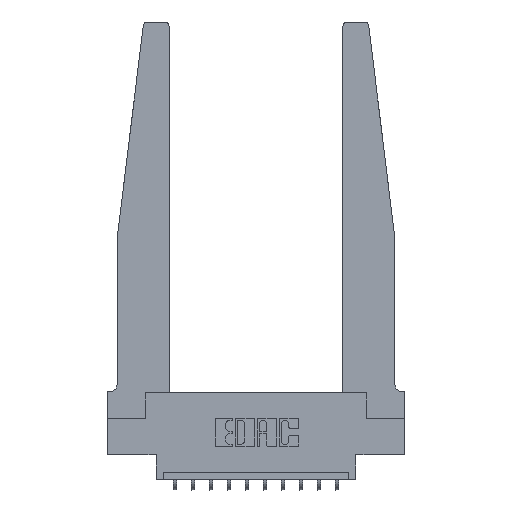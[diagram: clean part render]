
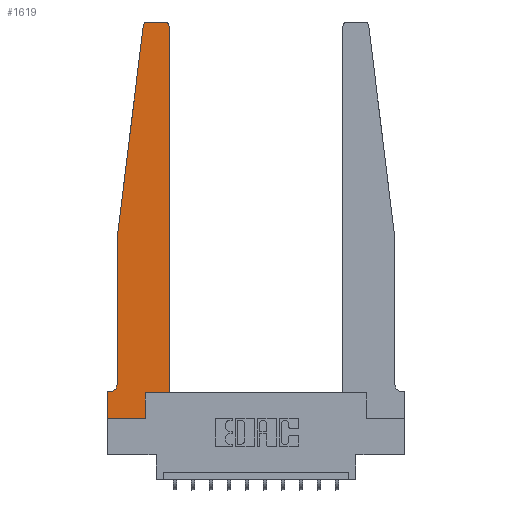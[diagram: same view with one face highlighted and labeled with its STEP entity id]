
A CAD part, top view. The second image highlights one B-rep face of the part: STEP entity #1619.
In plain terms, the highlighted planar face has unit normal (0, 0, 1).
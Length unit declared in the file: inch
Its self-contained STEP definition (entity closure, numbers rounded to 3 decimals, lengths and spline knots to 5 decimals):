
#219 = CARTESIAN_POINT ( 'NONE',  ( 0.015, 0.1875, 0.37 ) ) ;
#245 = DIRECTION ( 'NONE',  ( 0., 0., -1. ) ) ;
#351 = CARTESIAN_POINT ( 'NONE',  ( 0., 0.1875, 0.37 ) ) ;
#1283 = LINE ( 'NONE', #11136, #10915 ) ;
#1291 = VECTOR ( 'NONE', #9293, 39.37008 ) ;
#1331 = VERTEX_POINT ( 'NONE', #351 ) ;
#1425 = CARTESIAN_POINT ( 'NONE',  ( 0.065, 0.2375, 0.37 ) ) ;
#1446 = DIRECTION ( 'NONE',  ( -1., 0., 0. ) ) ;
#1536 = CARTESIAN_POINT ( 'NONE',  ( 0.425, 0.18, 0.37 ) ) ;
#1566 = DIRECTION ( 'NONE',  ( 0., 0., 1. ) ) ;
#1619 = ADVANCED_FACE ( 'NONE', ( #9924 ), #7503, .T. ) ;
#1737 = ORIENTED_EDGE ( 'NONE', *, *, #12814, .T. ) ;
#1752 = EDGE_CURVE ( 'NONE', #1331, #8008, #2641, .T. ) ;
#1868 = CARTESIAN_POINT ( 'NONE',  ( 0.065, 0.1875, 0.37 ) ) ;
#2068 = AXIS2_PLACEMENT_3D ( 'NONE', #9956, #1566, #6478 ) ;
#2637 = DIRECTION ( 'NONE',  ( 0., 1., 0. ) ) ;
#2641 = LINE ( 'NONE', #12758, #14164 ) ;
#2652 = LINE ( 'NONE', #6215, #13630 ) ;
#2748 = ORIENTED_EDGE ( 'NONE', *, *, #3446, .T. ) ;
#2854 = VECTOR ( 'NONE', #7429, 39.37008 ) ;
#2902 = CIRCLE ( 'NONE', #13999, 0.03 ) ;
#2942 = CARTESIAN_POINT ( 'NONE',  ( 0.2605, 0., 0.37 ) ) ;
#3031 = VERTEX_POINT ( 'NONE', #15523 ) ;
#3446 = EDGE_CURVE ( 'NONE', #14721, #13834, #15657, .T. ) ;
#3712 = CARTESIAN_POINT ( 'NONE',  ( 0., 0., 0.37 ) ) ;
#4086 = DIRECTION ( 'NONE',  ( -1., 0., 0. ) ) ;
#4157 = VECTOR ( 'NONE', #8885, 39.37008 ) ;
#4207 = EDGE_CURVE ( 'NONE', #13834, #12149, #9402, .T. ) ;
#4646 = CARTESIAN_POINT ( 'NONE',  ( 0.2605, 0.18, 0.37 ) ) ;
#4832 = DIRECTION ( 'NONE',  ( 1., 0., 0. ) ) ;
#4984 = DIRECTION ( 'NONE',  ( 1., 0., 0. ) ) ;
#5089 = EDGE_CURVE ( 'NONE', #6378, #12727, #10977, .T. ) ;
#5224 = CARTESIAN_POINT ( 'NONE',  ( 0.065, 1.25, 0.37 ) ) ;
#5264 = DIRECTION ( 'NONE',  ( 1., 0., 0. ) ) ;
#5334 = EDGE_CURVE ( 'NONE', #3031, #5651, #10321, .T. ) ;
#5345 = CARTESIAN_POINT ( 'NONE',  ( 0.395, 2.72, 0.37 ) ) ;
#5479 = LINE ( 'NONE', #7670, #4157 ) ;
#5651 = VERTEX_POINT ( 'NONE', #10226 ) ;
#5685 = CARTESIAN_POINT ( 'NONE',  ( 0.24675, 2.72367, 0.37 ) ) ;
#6155 = EDGE_LOOP ( 'NONE', ( #14824, #12152, #13387, #2748, #9065, #15544, #7193, #8934, #7471, #1737, #7129, #10539 ) ) ;
#6215 = CARTESIAN_POINT ( 'NONE',  ( 0.065, 1.25, 0.37 ) ) ;
#6341 = VECTOR ( 'NONE', #2637, 39.37008 ) ;
#6378 = VERTEX_POINT ( 'NONE', #13663 ) ;
#6478 = DIRECTION ( 'NONE',  ( 1., 0., 0. ) ) ;
#6559 = EDGE_CURVE ( 'NONE', #12727, #3031, #2902, .T. ) ;
#6861 = LINE ( 'NONE', #1868, #1291 ) ;
#6907 = EDGE_CURVE ( 'NONE', #15174, #8755, #5479, .T. ) ;
#6957 = CARTESIAN_POINT ( 'NONE',  ( 0.065, 1.25, 0.37 ) ) ;
#7062 = AXIS2_PLACEMENT_3D ( 'NONE', #7827, #245, #1446 ) ;
#7129 = ORIENTED_EDGE ( 'NONE', *, *, #5089, .T. ) ;
#7193 = ORIENTED_EDGE ( 'NONE', *, *, #1752, .T. ) ;
#7429 = DIRECTION ( 'NONE',  ( 1., 0., 0. ) ) ;
#7471 = ORIENTED_EDGE ( 'NONE', *, *, #6907, .T. ) ;
#7503 = PLANE ( 'NONE',  #14918 ) ;
#7670 = CARTESIAN_POINT ( 'NONE',  ( 0.2605, 0.18, 0.37 ) ) ;
#7827 = CARTESIAN_POINT ( 'NONE',  ( 0.015, 0.2375, 0.37 ) ) ;
#8008 = VERTEX_POINT ( 'NONE', #3712 ) ;
#8025 = EDGE_CURVE ( 'NONE', #15282, #14721, #2652, .T. ) ;
#8475 = DIRECTION ( 'NONE',  ( 0., 0., 1. ) ) ;
#8755 = VERTEX_POINT ( 'NONE', #4646 ) ;
#8792 = CARTESIAN_POINT ( 'NONE',  ( 0.425, 0.18, 0.37 ) ) ;
#8885 = DIRECTION ( 'NONE',  ( 0., 1., 0. ) ) ;
#8920 = VECTOR ( 'NONE', #13258, 39.37008 ) ;
#8934 = ORIENTED_EDGE ( 'NONE', *, *, #14763, .T. ) ;
#8953 = DIRECTION ( 'NONE',  ( 0., -1., 0. ) ) ;
#9065 = ORIENTED_EDGE ( 'NONE', *, *, #4207, .T. ) ;
#9229 = DIRECTION ( 'NONE',  ( 0., 0., 1. ) ) ;
#9293 = DIRECTION ( 'NONE',  ( -1., 0., 0. ) ) ;
#9343 = EDGE_CURVE ( 'NONE', #12149, #1331, #6861, .T. ) ;
#9378 = EDGE_CURVE ( 'NONE', #5651, #15282, #12636, .T. ) ;
#9402 = CIRCLE ( 'NONE', #7062, 0.05 ) ;
#9757 = CARTESIAN_POINT ( 'NONE',  ( 0., 0.1875, 0.37 ) ) ;
#9924 = FACE_OUTER_BOUND ( 'NONE', #6155, .T. ) ;
#9956 = CARTESIAN_POINT ( 'NONE',  ( 0.27653, 2.72, 0.37 ) ) ;
#10226 = CARTESIAN_POINT ( 'NONE',  ( 0.27653, 2.75, 0.37 ) ) ;
#10245 = CARTESIAN_POINT ( 'NONE',  ( 0.25, 2.75, 0.37 ) ) ;
#10321 = LINE ( 'NONE', #10245, #10719 ) ;
#10539 = ORIENTED_EDGE ( 'NONE', *, *, #6559, .T. ) ;
#10719 = VECTOR ( 'NONE', #4086, 39.37008 ) ;
#10915 = VECTOR ( 'NONE', #4984, 39.37008 ) ;
#10977 = LINE ( 'NONE', #8792, #6341 ) ;
#11136 = CARTESIAN_POINT ( 'NONE',  ( 0., 0., 0.37 ) ) ;
#12043 = CARTESIAN_POINT ( 'NONE',  ( 0.425, 2.72, 0.37 ) ) ;
#12149 = VERTEX_POINT ( 'NONE', #219 ) ;
#12152 = ORIENTED_EDGE ( 'NONE', *, *, #9378, .T. ) ;
#12285 = DIRECTION ( 'NONE',  ( -0.122, -0.992, 0. ) ) ;
#12360 = LINE ( 'NONE', #1536, #2854 ) ;
#12636 = CIRCLE ( 'NONE', #2068, 0.03 ) ;
#12727 = VERTEX_POINT ( 'NONE', #12043 ) ;
#12758 = CARTESIAN_POINT ( 'NONE',  ( 0., 0., 0.37 ) ) ;
#12814 = EDGE_CURVE ( 'NONE', #8755, #6378, #12360, .T. ) ;
#13258 = DIRECTION ( 'NONE',  ( 0., -1., 0. ) ) ;
#13387 = ORIENTED_EDGE ( 'NONE', *, *, #8025, .T. ) ;
#13630 = VECTOR ( 'NONE', #12285, 39.37008 ) ;
#13663 = CARTESIAN_POINT ( 'NONE',  ( 0.425, 0.18, 0.37 ) ) ;
#13834 = VERTEX_POINT ( 'NONE', #1425 ) ;
#13999 = AXIS2_PLACEMENT_3D ( 'NONE', #5345, #9229, #5264 ) ;
#14164 = VECTOR ( 'NONE', #8953, 39.37008 ) ;
#14721 = VERTEX_POINT ( 'NONE', #5224 ) ;
#14763 = EDGE_CURVE ( 'NONE', #8008, #15174, #1283, .T. ) ;
#14824 = ORIENTED_EDGE ( 'NONE', *, *, #5334, .T. ) ;
#14918 = AXIS2_PLACEMENT_3D ( 'NONE', #9757, #8475, #4832 ) ;
#15174 = VERTEX_POINT ( 'NONE', #2942 ) ;
#15282 = VERTEX_POINT ( 'NONE', #5685 ) ;
#15523 = CARTESIAN_POINT ( 'NONE',  ( 0.395, 2.75, 0.37 ) ) ;
#15544 = ORIENTED_EDGE ( 'NONE', *, *, #9343, .T. ) ;
#15657 = LINE ( 'NONE', #6957, #8920 ) ;
